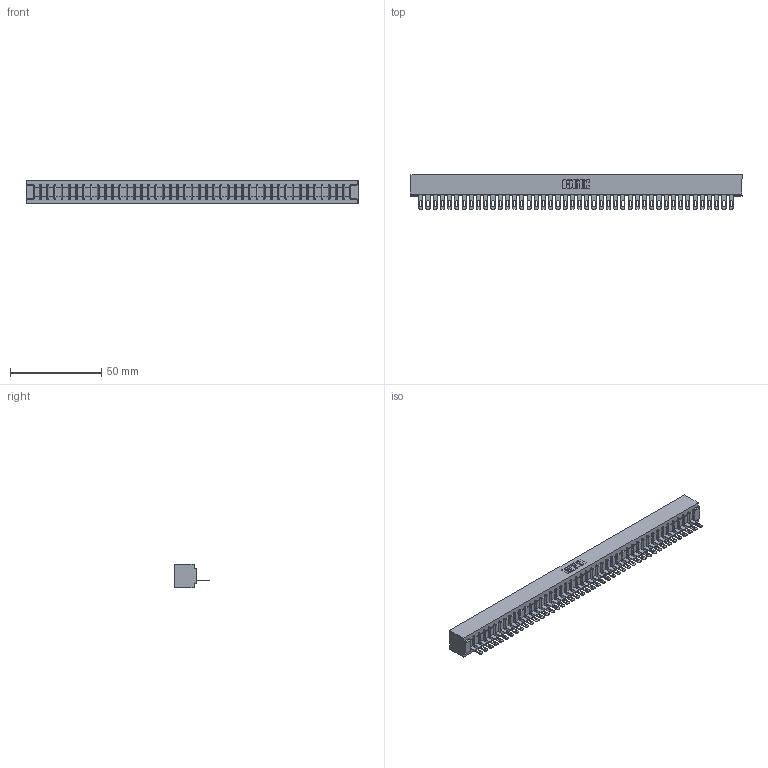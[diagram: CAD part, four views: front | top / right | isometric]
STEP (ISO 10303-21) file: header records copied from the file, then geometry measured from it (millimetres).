
FILE_DESCRIPTION (( 'STEP AP203' ), '1' );
FILE_NAME ('357-044-405-101.STEP', '2020-10-03T14:04:31', ( '' ), ( '' ), 'SwSTEP 2.0', 'SolidWorks 2020', '' );
FILE_SCHEMA (( 'CONFIG_CONTROL_DESIGN' ));
Length unit declared in the file: inch
Products named in the file (3): 357-044-405-101; 307-290-001_505; 307 Part_No Mounting Lugs
Assembly tree (45 placements, depth 2):
  357-044-405-101
    307 Part_No Mounting Lugs
    307-290-001_505  x44
Bounding box: 182.22 x 19.18 x 12.7 mm (x, y, z)
Volume: 19497 mm3; surface area: 21184.4 mm2
Topology: 45 solids, 45 shells, 2619 faces, 7427 edges, 4770 vertices
Faces by surface type: plane 1650, cylinder 879, sphere 90
Entity records: 37170 total; most frequent: CARTESIAN_POINT 6260, ORIENTED_EDGE 6246, DIRECTION 6087, EDGE_CURVE 3123, LINE 2397, VECTOR 2397, VERTEX_POINT 2018, AXIS2_PLACEMENT_3D 1845
